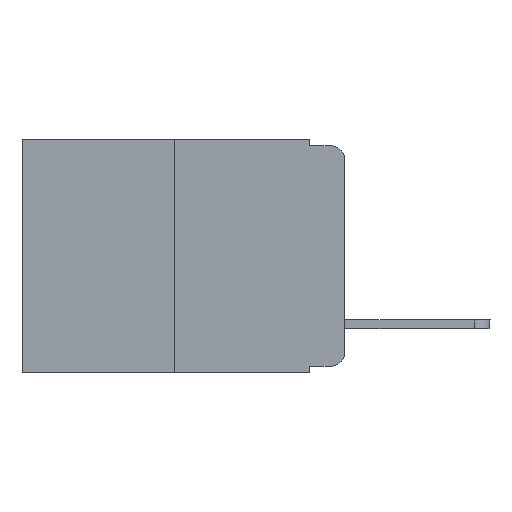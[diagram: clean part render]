
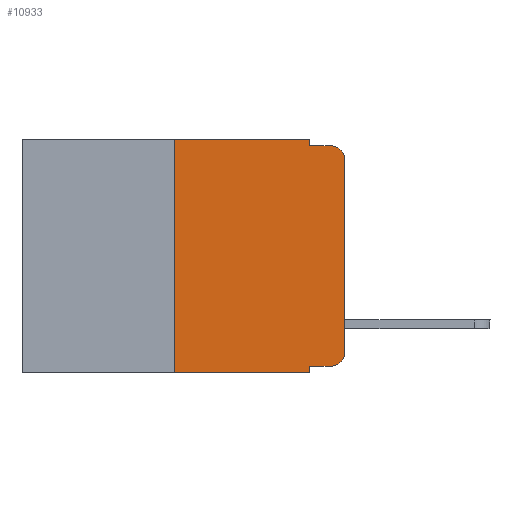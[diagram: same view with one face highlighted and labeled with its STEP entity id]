
A CAD part, left-side view. The second image highlights one B-rep face of the part: STEP entity #10933.
In plain terms, the highlighted planar face has unit normal (-1, 0, 0).
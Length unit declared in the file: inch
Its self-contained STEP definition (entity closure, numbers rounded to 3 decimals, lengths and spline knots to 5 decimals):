
#351 = DIRECTION ( 'NONE',  ( 0., 0., 1. ) ) ;
#670 = DIRECTION ( 'NONE',  ( 0., -1., 0. ) ) ;
#726 = ORIENTED_EDGE ( 'NONE', *, *, #8597, .T. ) ;
#1022 = ORIENTED_EDGE ( 'NONE', *, *, #5848, .F. ) ;
#1119 = VERTEX_POINT ( 'NONE', #10233 ) ;
#1225 = CIRCLE ( 'NONE', #11812, 0.02 ) ;
#1609 = CARTESIAN_POINT ( 'NONE',  ( 0., 0., -0.03 ) ) ;
#2206 = CARTESIAN_POINT ( 'NONE',  ( 0., 0.051, -0.01 ) ) ;
#2834 = VERTEX_POINT ( 'NONE', #1609 ) ;
#2884 = DIRECTION ( 'NONE',  ( 0., 0., -1. ) ) ;
#3578 = ORIENTED_EDGE ( 'NONE', *, *, #18973, .T. ) ;
#3958 = DIRECTION ( 'NONE',  ( 0., 0., 1. ) ) ;
#4112 = VERTEX_POINT ( 'NONE', #7053 ) ;
#4730 = VERTEX_POINT ( 'NONE', #11925 ) ;
#4751 = DIRECTION ( 'NONE',  ( -1., 0., 0. ) ) ;
#5073 = VERTEX_POINT ( 'NONE', #16244 ) ;
#5137 = CARTESIAN_POINT ( 'NONE',  ( 0., 0.051, 0. ) ) ;
#5848 = EDGE_CURVE ( 'NONE', #16335, #5073, #20240, .T. ) ;
#6105 = CARTESIAN_POINT ( 'NONE',  ( 0., 0., -0.313 ) ) ;
#6857 = LINE ( 'NONE', #13627, #7615 ) ;
#7053 = CARTESIAN_POINT ( 'NONE',  ( 0., 0.25, 0. ) ) ;
#7234 = CARTESIAN_POINT ( 'NONE',  ( 0., 0.02, -0.333 ) ) ;
#7308 = DIRECTION ( 'NONE',  ( 1., 0., 0. ) ) ;
#7506 = EDGE_CURVE ( 'NONE', #15091, #2834, #19587, .T. ) ;
#7522 = CARTESIAN_POINT ( 'NONE',  ( 0., 0.051, 0. ) ) ;
#7615 = VECTOR ( 'NONE', #3958, 39.37008 ) ;
#8457 = VERTEX_POINT ( 'NONE', #8668 ) ;
#8563 = VECTOR ( 'NONE', #670, 39.37008 ) ;
#8573 = VECTOR ( 'NONE', #2884, 39.37008 ) ;
#8597 = EDGE_CURVE ( 'NONE', #4730, #5073, #12130, .T. ) ;
#8668 = CARTESIAN_POINT ( 'NONE',  ( 0., 0.02, -0.01 ) ) ;
#9094 = CARTESIAN_POINT ( 'NONE',  ( 0., 0.02, -0.03 ) ) ;
#9493 = ORIENTED_EDGE ( 'NONE', *, *, #13276, .T. ) ;
#9612 = EDGE_CURVE ( 'NONE', #4112, #16641, #19268, .T. ) ;
#10081 = VECTOR ( 'NONE', #13233, 39.37008 ) ;
#10171 = ORIENTED_EDGE ( 'NONE', *, *, #7506, .T. ) ;
#10233 = CARTESIAN_POINT ( 'NONE',  ( 0., 0.051, -0.01 ) ) ;
#10856 = DIRECTION ( 'NONE',  ( 0., 0., -1. ) ) ;
#10933 = ADVANCED_FACE ( 'NONE', ( #20460 ), #17036, .F. ) ;
#11151 = CIRCLE ( 'NONE', #19377, 0.02 ) ;
#11726 = EDGE_LOOP ( 'NONE', ( #10171, #9493, #15537, #16005, #16616, #17660, #726, #1022, #16482, #3578 ) ) ;
#11812 = AXIS2_PLACEMENT_3D ( 'NONE', #17628, #4751, #10856 ) ;
#11925 = CARTESIAN_POINT ( 'NONE',  ( 0., 0.25, -0.343 ) ) ;
#12130 = LINE ( 'NONE', #17945, #10081 ) ;
#12350 = CARTESIAN_POINT ( 'NONE',  ( 0., 0.473, 0. ) ) ;
#12480 = EDGE_CURVE ( 'NONE', #1119, #8457, #15809, .T. ) ;
#13054 = EDGE_CURVE ( 'NONE', #4730, #4112, #6857, .T. ) ;
#13233 = DIRECTION ( 'NONE',  ( 0., -1., 0. ) ) ;
#13276 = EDGE_CURVE ( 'NONE', #2834, #8457, #11151, .T. ) ;
#13627 = CARTESIAN_POINT ( 'NONE',  ( 0., 0.25, 0. ) ) ;
#13781 = VERTEX_POINT ( 'NONE', #7234 ) ;
#13894 = LINE ( 'NONE', #7522, #8573 ) ;
#14260 = DIRECTION ( 'NONE',  ( 0., 0., -1. ) ) ;
#14547 = EDGE_CURVE ( 'NONE', #16641, #1119, #13894, .T. ) ;
#15019 = DIRECTION ( 'NONE',  ( 0., -1., 0. ) ) ;
#15091 = VERTEX_POINT ( 'NONE', #6105 ) ;
#15160 = CARTESIAN_POINT ( 'NONE',  ( 0., 0.473, 0. ) ) ;
#15161 = DIRECTION ( 'NONE',  ( 0., -1., 0. ) ) ;
#15232 = CARTESIAN_POINT ( 'NONE',  ( 0., 0.051, -0.333 ) ) ;
#15537 = ORIENTED_EDGE ( 'NONE', *, *, #12480, .F. ) ;
#15559 = DIRECTION ( 'NONE',  ( -1., 0., 0. ) ) ;
#15809 = LINE ( 'NONE', #2206, #17276 ) ;
#15824 = CARTESIAN_POINT ( 'NONE',  ( 0., 0.051, -0.333 ) ) ;
#15852 = LINE ( 'NONE', #15232, #16863 ) ;
#15902 = VECTOR ( 'NONE', #14260, 39.37008 ) ;
#16005 = ORIENTED_EDGE ( 'NONE', *, *, #14547, .F. ) ;
#16244 = CARTESIAN_POINT ( 'NONE',  ( 0., 0.051, -0.343 ) ) ;
#16335 = VERTEX_POINT ( 'NONE', #15824 ) ;
#16482 = ORIENTED_EDGE ( 'NONE', *, *, #20000, .T. ) ;
#16616 = ORIENTED_EDGE ( 'NONE', *, *, #9612, .F. ) ;
#16641 = VERTEX_POINT ( 'NONE', #5137 ) ;
#16682 = CARTESIAN_POINT ( 'NONE',  ( 0., 0., 0. ) ) ;
#16863 = VECTOR ( 'NONE', #15019, 39.37008 ) ;
#17036 = PLANE ( 'NONE',  #18102 ) ;
#17276 = VECTOR ( 'NONE', #15161, 39.37008 ) ;
#17628 = CARTESIAN_POINT ( 'NONE',  ( 0., 0.02, -0.313 ) ) ;
#17660 = ORIENTED_EDGE ( 'NONE', *, *, #13054, .F. ) ;
#17799 = VECTOR ( 'NONE', #351, 39.37008 ) ;
#17945 = CARTESIAN_POINT ( 'NONE',  ( 0., 0.473, -0.343 ) ) ;
#18102 = AXIS2_PLACEMENT_3D ( 'NONE', #12350, #7308, #18694 ) ;
#18694 = DIRECTION ( 'NONE',  ( 0., 0., -1. ) ) ;
#18973 = EDGE_CURVE ( 'NONE', #13781, #15091, #1225, .T. ) ;
#19268 = LINE ( 'NONE', #15160, #8563 ) ;
#19377 = AXIS2_PLACEMENT_3D ( 'NONE', #9094, #15559, #20480 ) ;
#19587 = LINE ( 'NONE', #16682, #17799 ) ;
#20000 = EDGE_CURVE ( 'NONE', #16335, #13781, #15852, .T. ) ;
#20240 = LINE ( 'NONE', #20467, #15902 ) ;
#20460 = FACE_OUTER_BOUND ( 'NONE', #11726, .T. ) ;
#20467 = CARTESIAN_POINT ( 'NONE',  ( 0., 0.051, 0. ) ) ;
#20480 = DIRECTION ( 'NONE',  ( 0., 0., -1. ) ) ;
